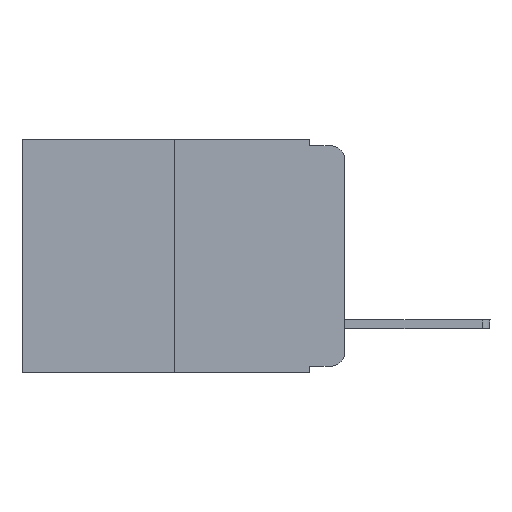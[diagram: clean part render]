
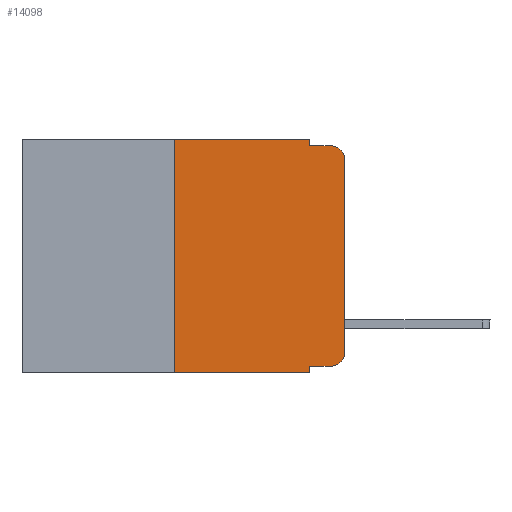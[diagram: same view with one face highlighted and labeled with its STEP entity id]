
A CAD part, left-side view. The second image highlights one B-rep face of the part: STEP entity #14098.
In plain terms, the highlighted planar face has unit normal (-1, 0, 0).
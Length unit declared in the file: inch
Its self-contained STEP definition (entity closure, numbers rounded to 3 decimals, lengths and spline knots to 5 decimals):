
#126 = CARTESIAN_POINT ( 'NONE',  ( 0., 0., -0.313 ) ) ;
#686 = LINE ( 'NONE', #17726, #13682 ) ;
#734 = DIRECTION ( 'NONE',  ( 0., 0., -1. ) ) ;
#973 = DIRECTION ( 'NONE',  ( 0., 0., -1. ) ) ;
#1405 = CARTESIAN_POINT ( 'NONE',  ( 0., 0.25, -0.343 ) ) ;
#1412 = DIRECTION ( 'NONE',  ( 1., 0., 0. ) ) ;
#1592 = EDGE_CURVE ( 'NONE', #7685, #19058, #3320, .T. ) ;
#2048 = ORIENTED_EDGE ( 'NONE', *, *, #6055, .F. ) ;
#2191 = EDGE_CURVE ( 'NONE', #17139, #4086, #4085, .T. ) ;
#2277 = CARTESIAN_POINT ( 'NONE',  ( 0., 0.25, 0. ) ) ;
#2425 = EDGE_CURVE ( 'NONE', #17139, #5015, #16103, .T. ) ;
#2825 = VECTOR ( 'NONE', #6700, 39.37008 ) ;
#3228 = CARTESIAN_POINT ( 'NONE',  ( 0., 0.051, 0. ) ) ;
#3320 = LINE ( 'NONE', #19124, #7240 ) ;
#3528 = DIRECTION ( 'NONE',  ( 0., 0., -1. ) ) ;
#4033 = CARTESIAN_POINT ( 'NONE',  ( 0., 0.473, -0.343 ) ) ;
#4085 = LINE ( 'NONE', #13361, #9668 ) ;
#4086 = VERTEX_POINT ( 'NONE', #19359 ) ;
#4134 = AXIS2_PLACEMENT_3D ( 'NONE', #8986, #1412, #12304 ) ;
#4449 = VECTOR ( 'NONE', #7970, 39.37008 ) ;
#4575 = ORIENTED_EDGE ( 'NONE', *, *, #18402, .F. ) ;
#4935 = EDGE_CURVE ( 'NONE', #5015, #8047, #6078, .T. ) ;
#5015 = VERTEX_POINT ( 'NONE', #11197 ) ;
#5173 = LINE ( 'NONE', #4033, #2825 ) ;
#6040 = CARTESIAN_POINT ( 'NONE',  ( 0., 0.02, -0.313 ) ) ;
#6055 = EDGE_CURVE ( 'NONE', #18792, #15282, #686, .T. ) ;
#6078 = CIRCLE ( 'NONE', #11335, 0.02 ) ;
#6120 = CARTESIAN_POINT ( 'NONE',  ( 0., 0., -0.03 ) ) ;
#6431 = CARTESIAN_POINT ( 'NONE',  ( 0., 0.051, -0.333 ) ) ;
#6700 = DIRECTION ( 'NONE',  ( 0., -1., 0. ) ) ;
#6913 = CIRCLE ( 'NONE', #11196, 0.02 ) ;
#7240 = VECTOR ( 'NONE', #3528, 39.37008 ) ;
#7308 = EDGE_LOOP ( 'NONE', ( #10633, #8912, #4575, #8542, #7494, #2048, #8199, #16860, #7357, #17779 ) ) ;
#7357 = ORIENTED_EDGE ( 'NONE', *, *, #2425, .T. ) ;
#7400 = EDGE_CURVE ( 'NONE', #8047, #10676, #8638, .T. ) ;
#7494 = ORIENTED_EDGE ( 'NONE', *, *, #18703, .F. ) ;
#7655 = PLANE ( 'NONE',  #4134 ) ;
#7685 = VERTEX_POINT ( 'NONE', #3228 ) ;
#7970 = DIRECTION ( 'NONE',  ( 0., -1., 0. ) ) ;
#8047 = VERTEX_POINT ( 'NONE', #126 ) ;
#8199 = ORIENTED_EDGE ( 'NONE', *, *, #16115, .T. ) ;
#8542 = ORIENTED_EDGE ( 'NONE', *, *, #1592, .F. ) ;
#8638 = LINE ( 'NONE', #16380, #11855 ) ;
#8912 = ORIENTED_EDGE ( 'NONE', *, *, #9157, .T. ) ;
#8986 = CARTESIAN_POINT ( 'NONE',  ( 0., 0.473, 0. ) ) ;
#9157 = EDGE_CURVE ( 'NONE', #10676, #15235, #6913, .T. ) ;
#9668 = VECTOR ( 'NONE', #734, 39.37008 ) ;
#10320 = CARTESIAN_POINT ( 'NONE',  ( 0., 0.473, 0. ) ) ;
#10633 = ORIENTED_EDGE ( 'NONE', *, *, #7400, .T. ) ;
#10676 = VERTEX_POINT ( 'NONE', #6120 ) ;
#11196 = AXIS2_PLACEMENT_3D ( 'NONE', #13340, #18350, #16490 ) ;
#11197 = CARTESIAN_POINT ( 'NONE',  ( 0., 0.02, -0.333 ) ) ;
#11335 = AXIS2_PLACEMENT_3D ( 'NONE', #6040, #18802, #973 ) ;
#11432 = CARTESIAN_POINT ( 'NONE',  ( 0., 0.02, -0.01 ) ) ;
#11855 = VECTOR ( 'NONE', #16174, 39.37008 ) ;
#11994 = LINE ( 'NONE', #10320, #12689 ) ;
#12304 = DIRECTION ( 'NONE',  ( 0., 0., -1. ) ) ;
#12689 = VECTOR ( 'NONE', #16487, 39.37008 ) ;
#12905 = CARTESIAN_POINT ( 'NONE',  ( 0., 0.051, -0.333 ) ) ;
#13340 = CARTESIAN_POINT ( 'NONE',  ( 0., 0.02, -0.03 ) ) ;
#13361 = CARTESIAN_POINT ( 'NONE',  ( 0., 0.051, 0. ) ) ;
#13682 = VECTOR ( 'NONE', #19553, 39.37008 ) ;
#13810 = CARTESIAN_POINT ( 'NONE',  ( 0., 0.051, -0.01 ) ) ;
#14098 = ADVANCED_FACE ( 'NONE', ( #18678 ), #7655, .F. ) ;
#14622 = VECTOR ( 'NONE', #15710, 39.37008 ) ;
#15235 = VERTEX_POINT ( 'NONE', #11432 ) ;
#15282 = VERTEX_POINT ( 'NONE', #2277 ) ;
#15710 = DIRECTION ( 'NONE',  ( 0., -1., 0. ) ) ;
#16103 = LINE ( 'NONE', #6431, #14622 ) ;
#16115 = EDGE_CURVE ( 'NONE', #18792, #4086, #5173, .T. ) ;
#16174 = DIRECTION ( 'NONE',  ( 0., 0., 1. ) ) ;
#16380 = CARTESIAN_POINT ( 'NONE',  ( 0., 0., 0. ) ) ;
#16487 = DIRECTION ( 'NONE',  ( 0., -1., 0. ) ) ;
#16490 = DIRECTION ( 'NONE',  ( 0., 0., -1. ) ) ;
#16860 = ORIENTED_EDGE ( 'NONE', *, *, #2191, .F. ) ;
#17139 = VERTEX_POINT ( 'NONE', #12905 ) ;
#17726 = CARTESIAN_POINT ( 'NONE',  ( 0., 0.25, 0. ) ) ;
#17779 = ORIENTED_EDGE ( 'NONE', *, *, #4935, .T. ) ;
#18350 = DIRECTION ( 'NONE',  ( -1., 0., 0. ) ) ;
#18402 = EDGE_CURVE ( 'NONE', #19058, #15235, #18471, .T. ) ;
#18471 = LINE ( 'NONE', #18582, #4449 ) ;
#18582 = CARTESIAN_POINT ( 'NONE',  ( 0., 0.051, -0.01 ) ) ;
#18678 = FACE_OUTER_BOUND ( 'NONE', #7308, .T. ) ;
#18703 = EDGE_CURVE ( 'NONE', #15282, #7685, #11994, .T. ) ;
#18792 = VERTEX_POINT ( 'NONE', #1405 ) ;
#18802 = DIRECTION ( 'NONE',  ( -1., 0., 0. ) ) ;
#19058 = VERTEX_POINT ( 'NONE', #13810 ) ;
#19124 = CARTESIAN_POINT ( 'NONE',  ( 0., 0.051, 0. ) ) ;
#19359 = CARTESIAN_POINT ( 'NONE',  ( 0., 0.051, -0.343 ) ) ;
#19553 = DIRECTION ( 'NONE',  ( 0., 0., 1. ) ) ;
